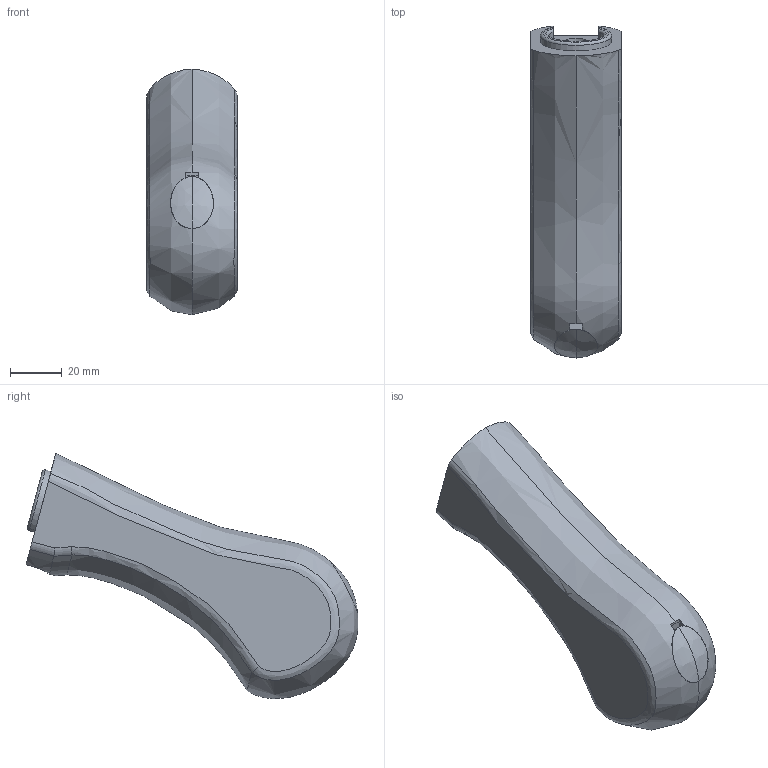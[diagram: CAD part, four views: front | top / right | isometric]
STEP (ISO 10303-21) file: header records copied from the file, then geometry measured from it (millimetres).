
FILE_DESCRIPTION(/* description */ (''),/* implementation_level */ '2;1');
FILE_NAME(/* name */ 'Birdshead Grip v2.step',/* time_stamp */ '2022-04-14T02:07:43-04:00',/* author */ (''),/* organization */ (''),/* preprocessor_version */ 'ST-DEVELOPER v18.1',/* originating_system */ 'Autodesk Translation Framework v10.14.0.1471',/* authorisation */ '');
FILE_SCHEMA (('AUTOMOTIVE_DESIGN { 1 0 10303 214 3 1 1 }'));
Length unit declared in the file: millimetre
Products named in the file (1): Birdshead Grip
Bounding box: 35.27 x 128.88 x 95.21 mm (x, y, z)
Volume: 163252.5 mm3; surface area: 26996.8 mm2
Topology: 3 solids, 3 shells, 54 faces, 139 edges, 92 vertices
Faces by surface type: plane 24, bspline 16, cylinder 12, torus 2
Full cylindrical faces by diameter (mm): 10 x2, 16.62 x1, 16.72 x1
Entity records: 3642 total; most frequent: CARTESIAN_POINT 2409, ORIENTED_EDGE 278, DIRECTION 194, EDGE_CURVE 139, VERTEX_POINT 92, AXIS2_PLACEMENT_3D 69, EDGE_LOOP 57, LINE 56
